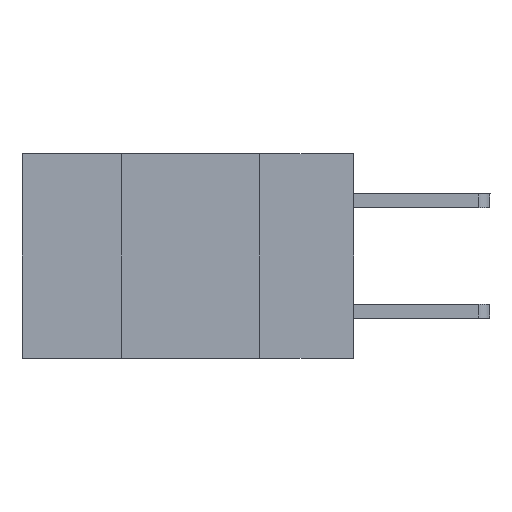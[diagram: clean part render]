
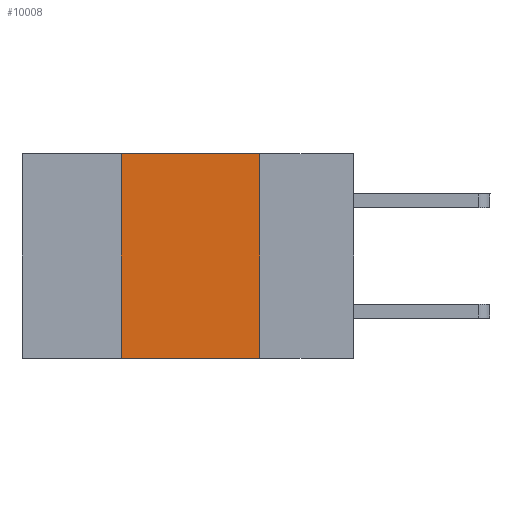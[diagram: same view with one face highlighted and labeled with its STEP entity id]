
A CAD part, left-side view. The second image highlights one B-rep face of the part: STEP entity #10008.
In plain terms, the highlighted planar face has unit normal (-1, 0, 0).
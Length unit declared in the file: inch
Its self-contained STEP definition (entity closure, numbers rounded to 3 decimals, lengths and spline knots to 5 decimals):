
#771 = LINE ( 'NONE', #1549, #9124 ) ;
#1351 = CARTESIAN_POINT ( 'NONE',  ( 0., 0.42, 0. ) ) ;
#1549 = CARTESIAN_POINT ( 'NONE',  ( 0., 0.17, 0. ) ) ;
#1660 = DIRECTION ( 'NONE',  ( 0., -1., 0. ) ) ;
#1795 = CARTESIAN_POINT ( 'NONE',  ( 0., 0.17, 0. ) ) ;
#2674 = ORIENTED_EDGE ( 'NONE', *, *, #5346, .F. ) ;
#3438 = CARTESIAN_POINT ( 'NONE',  ( 0., 0.42, -0.37 ) ) ;
#3802 = ORIENTED_EDGE ( 'NONE', *, *, #12367, .F. ) ;
#3835 = VERTEX_POINT ( 'NONE', #1795 ) ;
#3892 = VECTOR ( 'NONE', #10241, 39.37008 ) ;
#5117 = DIRECTION ( 'NONE',  ( 0., 0., -1. ) ) ;
#5346 = EDGE_CURVE ( 'NONE', #11534, #3835, #9947, .T. ) ;
#5401 = DIRECTION ( 'NONE',  ( 0., 0., -1. ) ) ;
#5442 = VECTOR ( 'NONE', #1660, 39.37008 ) ;
#5591 = CARTESIAN_POINT ( 'NONE',  ( 0., 0.6, 0. ) ) ;
#5623 = EDGE_CURVE ( 'NONE', #7171, #11534, #6056, .T. ) ;
#6007 = EDGE_LOOP ( 'NONE', ( #3802, #2674, #7138, #8864 ) ) ;
#6055 = FACE_OUTER_BOUND ( 'NONE', #6007, .T. ) ;
#6056 = LINE ( 'NONE', #9160, #3892 ) ;
#6440 = CARTESIAN_POINT ( 'NONE',  ( 0., 0.6, 0. ) ) ;
#7039 = DIRECTION ( 'NONE',  ( 0., -1., 0. ) ) ;
#7138 = ORIENTED_EDGE ( 'NONE', *, *, #5623, .F. ) ;
#7171 = VERTEX_POINT ( 'NONE', #3438 ) ;
#8864 = ORIENTED_EDGE ( 'NONE', *, *, #10717, .T. ) ;
#9124 = VECTOR ( 'NONE', #5401, 39.37008 ) ;
#9160 = CARTESIAN_POINT ( 'NONE',  ( 0., 0.42, 0. ) ) ;
#9169 = LINE ( 'NONE', #9882, #10212 ) ;
#9764 = PLANE ( 'NONE',  #9993 ) ;
#9882 = CARTESIAN_POINT ( 'NONE',  ( 0., 0.6, -0.37 ) ) ;
#9947 = LINE ( 'NONE', #6440, #5442 ) ;
#9993 = AXIS2_PLACEMENT_3D ( 'NONE', #5591, #10090, #5117 ) ;
#10008 = ADVANCED_FACE ( 'NONE', ( #6055 ), #9764, .F. ) ;
#10090 = DIRECTION ( 'NONE',  ( 1., 0., 0. ) ) ;
#10212 = VECTOR ( 'NONE', #7039, 39.37008 ) ;
#10241 = DIRECTION ( 'NONE',  ( 0., 0., 1. ) ) ;
#10717 = EDGE_CURVE ( 'NONE', #7171, #12508, #9169, .T. ) ;
#11534 = VERTEX_POINT ( 'NONE', #1351 ) ;
#12367 = EDGE_CURVE ( 'NONE', #3835, #12508, #771, .T. ) ;
#12508 = VERTEX_POINT ( 'NONE', #12574 ) ;
#12574 = CARTESIAN_POINT ( 'NONE',  ( 0., 0.17, -0.37 ) ) ;
